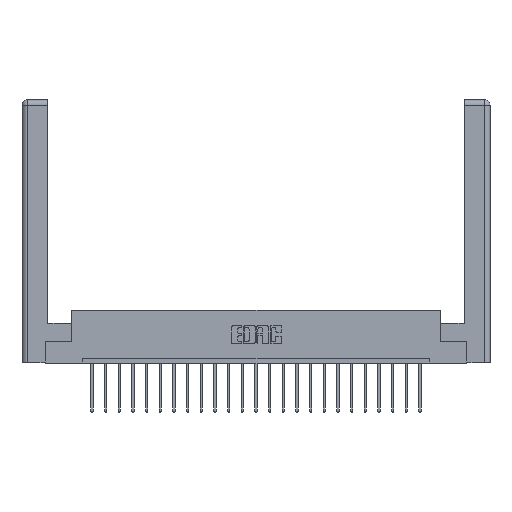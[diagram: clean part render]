
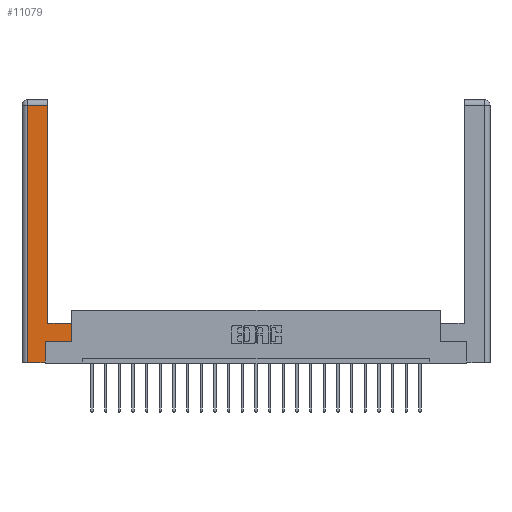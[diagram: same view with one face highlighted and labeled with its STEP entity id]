
A CAD part, top view. The second image highlights one B-rep face of the part: STEP entity #11079.
In plain terms, the highlighted planar face has unit normal (0, 0, 1).
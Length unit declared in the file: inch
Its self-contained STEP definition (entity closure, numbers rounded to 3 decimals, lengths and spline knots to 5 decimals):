
#53 = EDGE_CURVE ( 'NONE', #6812, #15490, #7628, .T. ) ;
#624 = CARTESIAN_POINT ( 'NONE',  ( 0.295, 0.45, 0. ) ) ;
#773 = DIRECTION ( 'NONE',  ( 0., 0., -1. ) ) ;
#806 = PLANE ( 'NONE',  #15000 ) ;
#1244 = DIRECTION ( 'NONE',  ( 0., 1., 0. ) ) ;
#1435 = VECTOR ( 'NONE', #9565, 39.37008 ) ;
#1485 = LINE ( 'NONE', #3297, #14225 ) ;
#1490 = ORIENTED_EDGE ( 'NONE', *, *, #9606, .T. ) ;
#2498 = EDGE_CURVE ( 'NONE', #2971, #21096, #7373, .T. ) ;
#2971 = VERTEX_POINT ( 'NONE', #12616 ) ;
#3297 = CARTESIAN_POINT ( 'NONE',  ( 0.565, 0.45, 0. ) ) ;
#4049 = EDGE_CURVE ( 'NONE', #17536, #16087, #8155, .T. ) ;
#4474 = CARTESIAN_POINT ( 'NONE',  ( 0.565, 0.245, 0. ) ) ;
#5126 = EDGE_CURVE ( 'NONE', #8127, #17536, #19176, .T. ) ;
#5368 = CARTESIAN_POINT ( 'NONE',  ( 0.295, 2.94, 0. ) ) ;
#5934 = CARTESIAN_POINT ( 'NONE',  ( 0., 0., 0. ) ) ;
#6349 = DIRECTION ( 'NONE',  ( 1., 0., 0. ) ) ;
#6715 = CARTESIAN_POINT ( 'NONE',  ( 0.0615, 0., 0. ) ) ;
#6812 = VERTEX_POINT ( 'NONE', #14121 ) ;
#6907 = DIRECTION ( 'NONE',  ( 0., 1., 0. ) ) ;
#7288 = VECTOR ( 'NONE', #1244, 39.37008 ) ;
#7373 = LINE ( 'NONE', #11773, #9657 ) ;
#7628 = LINE ( 'NONE', #4474, #1435 ) ;
#7895 = ORIENTED_EDGE ( 'NONE', *, *, #13944, .T. ) ;
#8127 = VERTEX_POINT ( 'NONE', #12069 ) ;
#8155 = LINE ( 'NONE', #11818, #23193 ) ;
#8754 = ORIENTED_EDGE ( 'NONE', *, *, #2498, .T. ) ;
#8879 = VECTOR ( 'NONE', #13736, 39.37008 ) ;
#9514 = VERTEX_POINT ( 'NONE', #15678 ) ;
#9565 = DIRECTION ( 'NONE',  ( 1., 0., 0. ) ) ;
#9606 = EDGE_CURVE ( 'NONE', #21096, #6812, #21887, .T. ) ;
#9657 = VECTOR ( 'NONE', #6349, 39.37008 ) ;
#10035 = LINE ( 'NONE', #624, #16830 ) ;
#10082 = EDGE_CURVE ( 'NONE', #15490, #9514, #1485, .T. ) ;
#10306 = FACE_OUTER_BOUND ( 'NONE', #16313, .T. ) ;
#10470 = ORIENTED_EDGE ( 'NONE', *, *, #53, .T. ) ;
#11079 = ADVANCED_FACE ( 'NONE', ( #10306 ), #806, .F. ) ;
#11773 = CARTESIAN_POINT ( 'NONE',  ( 0.265, 0., 0. ) ) ;
#11818 = CARTESIAN_POINT ( 'NONE',  ( 0.0615, 2.94, 0. ) ) ;
#12069 = CARTESIAN_POINT ( 'NONE',  ( 0.295, 0.45, 0. ) ) ;
#12616 = CARTESIAN_POINT ( 'NONE',  ( 0.0615, 0., 0. ) ) ;
#13189 = EDGE_CURVE ( 'NONE', #16087, #2971, #18967, .T. ) ;
#13709 = DIRECTION ( 'NONE',  ( -1., 0., 0. ) ) ;
#13736 = DIRECTION ( 'NONE',  ( 0., 1., 0. ) ) ;
#13944 = EDGE_CURVE ( 'NONE', #9514, #8127, #10035, .T. ) ;
#13963 = CARTESIAN_POINT ( 'NONE',  ( 0.0615, 2.94, 0. ) ) ;
#14121 = CARTESIAN_POINT ( 'NONE',  ( 0.265, 0.245, 0. ) ) ;
#14150 = CARTESIAN_POINT ( 'NONE',  ( 0.295, 3., 0. ) ) ;
#14225 = VECTOR ( 'NONE', #6907, 39.37008 ) ;
#15000 = AXIS2_PLACEMENT_3D ( 'NONE', #5934, #773, #18958 ) ;
#15490 = VERTEX_POINT ( 'NONE', #19942 ) ;
#15678 = CARTESIAN_POINT ( 'NONE',  ( 0.565, 0.45, 0. ) ) ;
#15774 = CARTESIAN_POINT ( 'NONE',  ( 0.265, 0., 0. ) ) ;
#16087 = VERTEX_POINT ( 'NONE', #13963 ) ;
#16313 = EDGE_LOOP ( 'NONE', ( #18226, #16949, #20808, #8754, #1490, #10470, #19075, #7895 ) ) ;
#16830 = VECTOR ( 'NONE', #18353, 39.37008 ) ;
#16949 = ORIENTED_EDGE ( 'NONE', *, *, #4049, .T. ) ;
#17536 = VERTEX_POINT ( 'NONE', #5368 ) ;
#17668 = DIRECTION ( 'NONE',  ( 0., -1., 0. ) ) ;
#17854 = VECTOR ( 'NONE', #17668, 39.37008 ) ;
#18226 = ORIENTED_EDGE ( 'NONE', *, *, #5126, .T. ) ;
#18353 = DIRECTION ( 'NONE',  ( -1., 0., 0. ) ) ;
#18958 = DIRECTION ( 'NONE',  ( -1., 0., 0. ) ) ;
#18967 = LINE ( 'NONE', #6715, #17854 ) ;
#19075 = ORIENTED_EDGE ( 'NONE', *, *, #10082, .T. ) ;
#19176 = LINE ( 'NONE', #14150, #7288 ) ;
#19418 = CARTESIAN_POINT ( 'NONE',  ( 0.265, 0.245, 0. ) ) ;
#19942 = CARTESIAN_POINT ( 'NONE',  ( 0.565, 0.245, 0. ) ) ;
#20808 = ORIENTED_EDGE ( 'NONE', *, *, #13189, .T. ) ;
#21096 = VERTEX_POINT ( 'NONE', #15774 ) ;
#21887 = LINE ( 'NONE', #19418, #8879 ) ;
#23193 = VECTOR ( 'NONE', #13709, 39.37008 ) ;
